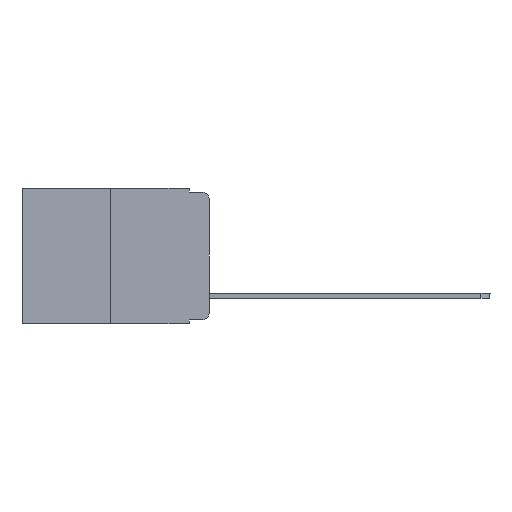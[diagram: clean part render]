
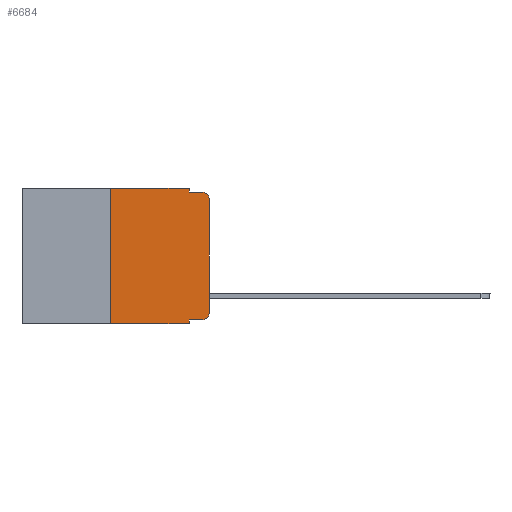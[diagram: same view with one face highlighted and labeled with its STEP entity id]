
A CAD part, left-side view. The second image highlights one B-rep face of the part: STEP entity #6684.
In plain terms, the highlighted planar face has unit normal (-1, 0, 0).
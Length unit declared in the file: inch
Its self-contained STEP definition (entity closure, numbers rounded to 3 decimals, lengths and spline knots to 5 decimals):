
#72 = CARTESIAN_POINT ( 'NONE',  ( 0., 0.02, -0.01 ) ) ;
#201 = EDGE_CURVE ( 'NONE', #1834, #8995, #6855, .T. ) ;
#223 = AXIS2_PLACEMENT_3D ( 'NONE', #9707, #1749, #8917 ) ;
#240 = VECTOR ( 'NONE', #3728, 39.37008 ) ;
#307 = LINE ( 'NONE', #3480, #7778 ) ;
#321 = DIRECTION ( 'NONE',  ( 0., -1., 0. ) ) ;
#420 = EDGE_CURVE ( 'NONE', #8995, #5634, #6031, .T. ) ;
#476 = CARTESIAN_POINT ( 'NONE',  ( 0., 0.473, 0. ) ) ;
#644 = CARTESIAN_POINT ( 'NONE',  ( 0., 0.051, 0. ) ) ;
#656 = LINE ( 'NONE', #6176, #240 ) ;
#775 = CARTESIAN_POINT ( 'NONE',  ( 0., 0.051, 0. ) ) ;
#789 = VECTOR ( 'NONE', #321, 39.37008 ) ;
#816 = CIRCLE ( 'NONE', #9311, 0.02 ) ;
#1255 = DIRECTION ( 'NONE',  ( 0., -1., 0. ) ) ;
#1367 = EDGE_LOOP ( 'NONE', ( #4774, #9857, #5679, #8022, #3082, #3367, #1595, #7475, #8542, #6268 ) ) ;
#1393 = AXIS2_PLACEMENT_3D ( 'NONE', #2264, #5411, #1472 ) ;
#1472 = DIRECTION ( 'NONE',  ( 0., 0., -1. ) ) ;
#1500 = CARTESIAN_POINT ( 'NONE',  ( 0., 0., -0.313 ) ) ;
#1595 = ORIENTED_EDGE ( 'NONE', *, *, #6628, .T. ) ;
#1726 = VECTOR ( 'NONE', #9939, 39.37008 ) ;
#1749 = DIRECTION ( 'NONE',  ( 1., 0., 0. ) ) ;
#1795 = VERTEX_POINT ( 'NONE', #9478 ) ;
#1828 = CARTESIAN_POINT ( 'NONE',  ( 0., 0., -0.03 ) ) ;
#1834 = VERTEX_POINT ( 'NONE', #2540 ) ;
#1839 = LINE ( 'NONE', #6046, #789 ) ;
#1964 = EDGE_CURVE ( 'NONE', #1795, #1834, #307, .T. ) ;
#2219 = VECTOR ( 'NONE', #1255, 39.37008 ) ;
#2264 = CARTESIAN_POINT ( 'NONE',  ( 0., 0.02, -0.313 ) ) ;
#2442 = VERTEX_POINT ( 'NONE', #6105 ) ;
#2540 = CARTESIAN_POINT ( 'NONE',  ( 0., 0.02, -0.333 ) ) ;
#2851 = VERTEX_POINT ( 'NONE', #8758 ) ;
#3082 = ORIENTED_EDGE ( 'NONE', *, *, #8588, .F. ) ;
#3353 = VERTEX_POINT ( 'NONE', #72 ) ;
#3367 = ORIENTED_EDGE ( 'NONE', *, *, #7655, .F. ) ;
#3388 = CARTESIAN_POINT ( 'NONE',  ( 0., 0.02, -0.03 ) ) ;
#3464 = CARTESIAN_POINT ( 'NONE',  ( 0., 0.25, 0. ) ) ;
#3480 = CARTESIAN_POINT ( 'NONE',  ( 0., 0.051, -0.333 ) ) ;
#3728 = DIRECTION ( 'NONE',  ( 0., 0., 1. ) ) ;
#3757 = DIRECTION ( 'NONE',  ( 0., -1., 0. ) ) ;
#3780 = CARTESIAN_POINT ( 'NONE',  ( 0., 0.051, 0. ) ) ;
#3953 = DIRECTION ( 'NONE',  ( 0., 0., -1. ) ) ;
#4152 = VECTOR ( 'NONE', #6023, 39.37008 ) ;
#4291 = EDGE_CURVE ( 'NONE', #1795, #2442, #4934, .T. ) ;
#4470 = EDGE_CURVE ( 'NONE', #9454, #5361, #5173, .T. ) ;
#4774 = ORIENTED_EDGE ( 'NONE', *, *, #420, .T. ) ;
#4934 = LINE ( 'NONE', #775, #10196 ) ;
#5173 = LINE ( 'NONE', #3780, #4152 ) ;
#5361 = VERTEX_POINT ( 'NONE', #7683 ) ;
#5411 = DIRECTION ( 'NONE',  ( -1., 0., 0. ) ) ;
#5634 = VERTEX_POINT ( 'NONE', #1828 ) ;
#5679 = ORIENTED_EDGE ( 'NONE', *, *, #6504, .F. ) ;
#6023 = DIRECTION ( 'NONE',  ( 0., 0., -1. ) ) ;
#6031 = LINE ( 'NONE', #9207, #1726 ) ;
#6046 = CARTESIAN_POINT ( 'NONE',  ( 0., 0.051, -0.01 ) ) ;
#6105 = CARTESIAN_POINT ( 'NONE',  ( 0., 0.051, -0.343 ) ) ;
#6176 = CARTESIAN_POINT ( 'NONE',  ( 0., 0.25, 0. ) ) ;
#6268 = ORIENTED_EDGE ( 'NONE', *, *, #201, .T. ) ;
#6448 = EDGE_CURVE ( 'NONE', #5634, #3353, #816, .T. ) ;
#6504 = EDGE_CURVE ( 'NONE', #5361, #3353, #1839, .T. ) ;
#6628 = EDGE_CURVE ( 'NONE', #2851, #2442, #9177, .T. ) ;
#6647 = DIRECTION ( 'NONE',  ( 0., -1., 0. ) ) ;
#6684 = ADVANCED_FACE ( 'NONE', ( #9770 ), #9660, .F. ) ;
#6711 = CARTESIAN_POINT ( 'NONE',  ( 0., 0.473, -0.343 ) ) ;
#6855 = CIRCLE ( 'NONE', #1393, 0.02 ) ;
#6866 = LINE ( 'NONE', #476, #7205 ) ;
#7205 = VECTOR ( 'NONE', #3757, 39.37008 ) ;
#7475 = ORIENTED_EDGE ( 'NONE', *, *, #4291, .F. ) ;
#7655 = EDGE_CURVE ( 'NONE', #2851, #8046, #656, .T. ) ;
#7683 = CARTESIAN_POINT ( 'NONE',  ( 0., 0.051, -0.01 ) ) ;
#7778 = VECTOR ( 'NONE', #6647, 39.37008 ) ;
#8022 = ORIENTED_EDGE ( 'NONE', *, *, #4470, .F. ) ;
#8046 = VERTEX_POINT ( 'NONE', #3464 ) ;
#8210 = DIRECTION ( 'NONE',  ( 0., 0., -1. ) ) ;
#8542 = ORIENTED_EDGE ( 'NONE', *, *, #1964, .T. ) ;
#8588 = EDGE_CURVE ( 'NONE', #8046, #9454, #6866, .T. ) ;
#8758 = CARTESIAN_POINT ( 'NONE',  ( 0., 0.25, -0.343 ) ) ;
#8917 = DIRECTION ( 'NONE',  ( 0., 0., -1. ) ) ;
#8995 = VERTEX_POINT ( 'NONE', #1500 ) ;
#9012 = DIRECTION ( 'NONE',  ( -1., 0., 0. ) ) ;
#9177 = LINE ( 'NONE', #6711, #2219 ) ;
#9207 = CARTESIAN_POINT ( 'NONE',  ( 0., 0., 0. ) ) ;
#9311 = AXIS2_PLACEMENT_3D ( 'NONE', #3388, #9012, #8210 ) ;
#9454 = VERTEX_POINT ( 'NONE', #644 ) ;
#9478 = CARTESIAN_POINT ( 'NONE',  ( 0., 0.051, -0.333 ) ) ;
#9660 = PLANE ( 'NONE',  #223 ) ;
#9707 = CARTESIAN_POINT ( 'NONE',  ( 0., 0.473, 0. ) ) ;
#9770 = FACE_OUTER_BOUND ( 'NONE', #1367, .T. ) ;
#9857 = ORIENTED_EDGE ( 'NONE', *, *, #6448, .T. ) ;
#9939 = DIRECTION ( 'NONE',  ( 0., 0., 1. ) ) ;
#10196 = VECTOR ( 'NONE', #3953, 39.37008 ) ;
